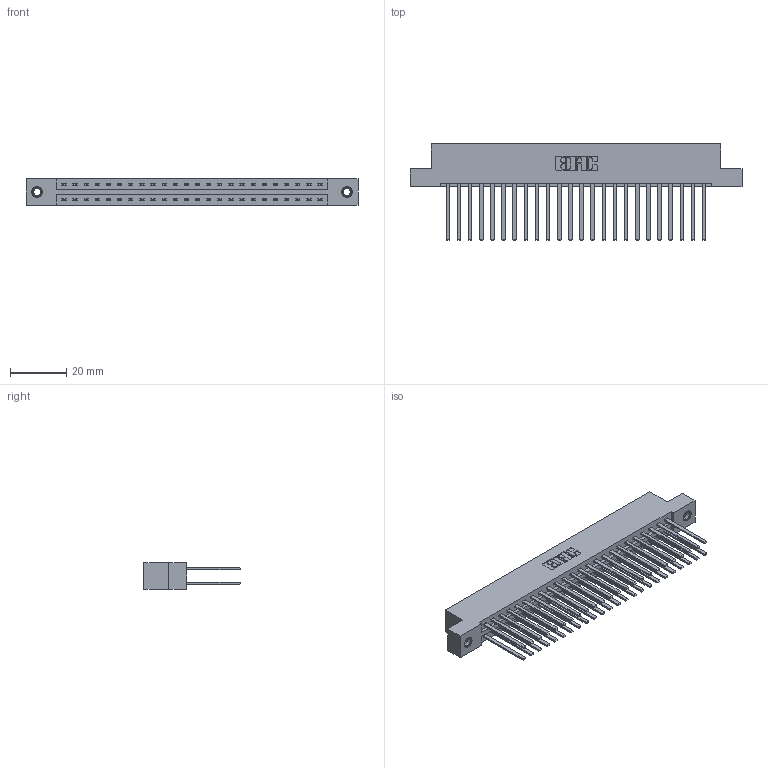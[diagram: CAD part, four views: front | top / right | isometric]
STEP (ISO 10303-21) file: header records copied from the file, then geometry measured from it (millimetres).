
FILE_DESCRIPTION (( 'STEP AP203' ), '1' );
FILE_NAME ('387-048-544-207.STEP', '2019-10-18T10:09:26', ( '' ), ( '' ), 'SwSTEP 2.0', 'SolidWorks 2016', '' );
FILE_SCHEMA (( 'CONFIG_CONTROL_DESIGN' ));
Length unit declared in the file: inch
Products named in the file (4): 345-292-001_345-293-144; 337 Part_Flush Mounting Lugs - 0.156 Dia-TI; 387-048-544-207; 345-250-001_345-250-005-103
Assembly tree (51 placements, depth 2):
  387-048-544-207
    337 Part_Flush Mounting Lugs - 0.156 Dia-TI
    345-292-001_345-293-144  x48
    345-250-001_345-250-005-103  x2
Bounding box: 118.11 x 34.3 x 9.4 mm (x, y, z)
Volume: 12867.1 mm3; surface area: 16605.5 mm2
Topology: 51 solids, 51 shells, 2478 faces, 7311 edges, 4802 vertices
Faces by surface type: plane 1734, cylinder 728, cone 12, torus 4
Entity records: 21938 total; most frequent: CARTESIAN_POINT 3689, ORIENTED_EDGE 3618, DIRECTION 3199, EDGE_CURVE 1809, LINE 1665, VECTOR 1665, VERTEX_POINT 1200, AXIS2_PLACEMENT_3D 767
